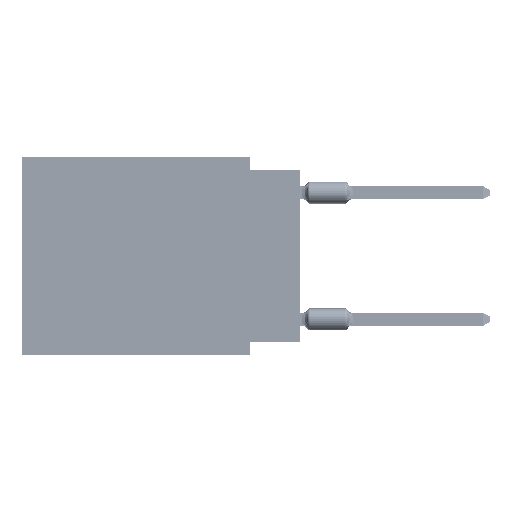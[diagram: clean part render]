
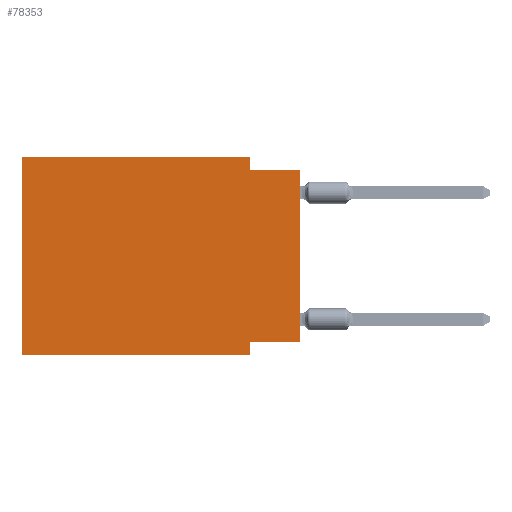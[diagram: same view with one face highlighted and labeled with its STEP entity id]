
A CAD part, left-side view. The second image highlights one B-rep face of the part: STEP entity #78353.
In plain terms, the highlighted planar face has unit normal (-1, 0, 0).
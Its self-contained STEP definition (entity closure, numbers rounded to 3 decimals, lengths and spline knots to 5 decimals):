
#1410 = EDGE_CURVE ( 'NONE', #22567, #60050, #23946, .T. ) ;
#4293 = CARTESIAN_POINT ( 'NONE',  ( 0., 0.55, 0. ) ) ;
#8976 = CARTESIAN_POINT ( 'NONE',  ( 0., 0., -0.025 ) ) ;
#9484 = DIRECTION ( 'NONE',  ( 0., -1., 0. ) ) ;
#10373 = VECTOR ( 'NONE', #34190, 39.37008 ) ;
#11281 = ORIENTED_EDGE ( 'NONE', *, *, #24983, .F. ) ;
#13660 = LINE ( 'NONE', #45730, #56316 ) ;
#13687 = EDGE_CURVE ( 'NONE', #15252, #24128, #78204, .T. ) ;
#14317 = PLANE ( 'NONE',  #30656 ) ;
#14470 = VERTEX_POINT ( 'NONE', #70643 ) ;
#15252 = VERTEX_POINT ( 'NONE', #75601 ) ;
#16025 = DIRECTION ( 'NONE',  ( 0., 0., -1. ) ) ;
#17541 = DIRECTION ( 'NONE',  ( 0., -1., 0. ) ) ;
#17838 = VECTOR ( 'NONE', #20885, 39.37008 ) ;
#20885 = DIRECTION ( 'NONE',  ( 0., 1., 0. ) ) ;
#21441 = DIRECTION ( 'NONE',  ( 0., 0., -1. ) ) ;
#22567 = VERTEX_POINT ( 'NONE', #47158 ) ;
#23946 = LINE ( 'NONE', #4293, #41356 ) ;
#24128 = VERTEX_POINT ( 'NONE', #32568 ) ;
#24983 = EDGE_CURVE ( 'NONE', #60050, #78683, #48087, .T. ) ;
#25753 = VERTEX_POINT ( 'NONE', #40944 ) ;
#25902 = LINE ( 'NONE', #51980, #51563 ) ;
#30334 = VERTEX_POINT ( 'NONE', #60160 ) ;
#30656 = AXIS2_PLACEMENT_3D ( 'NONE', #39955, #72460, #78872 ) ;
#31697 = EDGE_CURVE ( 'NONE', #15252, #30334, #25902, .T. ) ;
#32568 = CARTESIAN_POINT ( 'NONE',  ( 0., 0.1, -0.365 ) ) ;
#32812 = ORIENTED_EDGE ( 'NONE', *, *, #82016, .F. ) ;
#34190 = DIRECTION ( 'NONE',  ( 0., -1., 0. ) ) ;
#36749 = ORIENTED_EDGE ( 'NONE', *, *, #31697, .T. ) ;
#36811 = LINE ( 'NONE', #54383, #82019 ) ;
#37921 = VECTOR ( 'NONE', #21441, 39.37008 ) ;
#39955 = CARTESIAN_POINT ( 'NONE',  ( 0., 0.55, 0. ) ) ;
#40944 = CARTESIAN_POINT ( 'NONE',  ( 0., 0.1, -0.39 ) ) ;
#41356 = VECTOR ( 'NONE', #17541, 39.37008 ) ;
#45527 = EDGE_CURVE ( 'NONE', #24128, #25753, #65509, .T. ) ;
#45730 = CARTESIAN_POINT ( 'NONE',  ( 0., 0.55, 0. ) ) ;
#45841 = CARTESIAN_POINT ( 'NONE',  ( 0., 0.1, -0.39 ) ) ;
#46873 = EDGE_CURVE ( 'NONE', #14470, #25753, #36811, .T. ) ;
#47158 = CARTESIAN_POINT ( 'NONE',  ( 0., 0.55, 0. ) ) ;
#47764 = ORIENTED_EDGE ( 'NONE', *, *, #46873, .T. ) ;
#48087 = LINE ( 'NONE', #54501, #52428 ) ;
#50580 = CARTESIAN_POINT ( 'NONE',  ( 0., 0.1, -0.025 ) ) ;
#51563 = VECTOR ( 'NONE', #71656, 39.37008 ) ;
#51980 = CARTESIAN_POINT ( 'NONE',  ( 0., 0., 0. ) ) ;
#52144 = DIRECTION ( 'NONE',  ( 0., 0., 1. ) ) ;
#52428 = VECTOR ( 'NONE', #16025, 39.37008 ) ;
#54383 = CARTESIAN_POINT ( 'NONE',  ( 0., 0.55, -0.39 ) ) ;
#54501 = CARTESIAN_POINT ( 'NONE',  ( 0., 0.1, 0. ) ) ;
#54697 = LINE ( 'NONE', #8976, #10373 ) ;
#56316 = VECTOR ( 'NONE', #52144, 39.37008 ) ;
#56566 = EDGE_LOOP ( 'NONE', ( #36749, #32812, #11281, #69751, #75031, #47764, #78162, #72427 ) ) ;
#60050 = VERTEX_POINT ( 'NONE', #69646 ) ;
#60160 = CARTESIAN_POINT ( 'NONE',  ( 0., 0., -0.025 ) ) ;
#63575 = EDGE_CURVE ( 'NONE', #14470, #22567, #13660, .T. ) ;
#65509 = LINE ( 'NONE', #45841, #37921 ) ;
#69646 = CARTESIAN_POINT ( 'NONE',  ( 0., 0.1, 0. ) ) ;
#69751 = ORIENTED_EDGE ( 'NONE', *, *, #1410, .F. ) ;
#70643 = CARTESIAN_POINT ( 'NONE',  ( 0., 0.55, -0.39 ) ) ;
#71375 = CARTESIAN_POINT ( 'NONE',  ( 0., 0., -0.365 ) ) ;
#71656 = DIRECTION ( 'NONE',  ( 0., 0., 1. ) ) ;
#72427 = ORIENTED_EDGE ( 'NONE', *, *, #13687, .F. ) ;
#72460 = DIRECTION ( 'NONE',  ( 1., 0., 0. ) ) ;
#75031 = ORIENTED_EDGE ( 'NONE', *, *, #63575, .F. ) ;
#75601 = CARTESIAN_POINT ( 'NONE',  ( 0., 0., -0.365 ) ) ;
#78017 = FACE_OUTER_BOUND ( 'NONE', #56566, .T. ) ;
#78162 = ORIENTED_EDGE ( 'NONE', *, *, #45527, .F. ) ;
#78204 = LINE ( 'NONE', #71375, #17838 ) ;
#78353 = ADVANCED_FACE ( 'NONE', ( #78017 ), #14317, .F. ) ;
#78683 = VERTEX_POINT ( 'NONE', #50580 ) ;
#78872 = DIRECTION ( 'NONE',  ( 0., 0., -1. ) ) ;
#82016 = EDGE_CURVE ( 'NONE', #78683, #30334, #54697, .T. ) ;
#82019 = VECTOR ( 'NONE', #9484, 39.37008 ) ;
